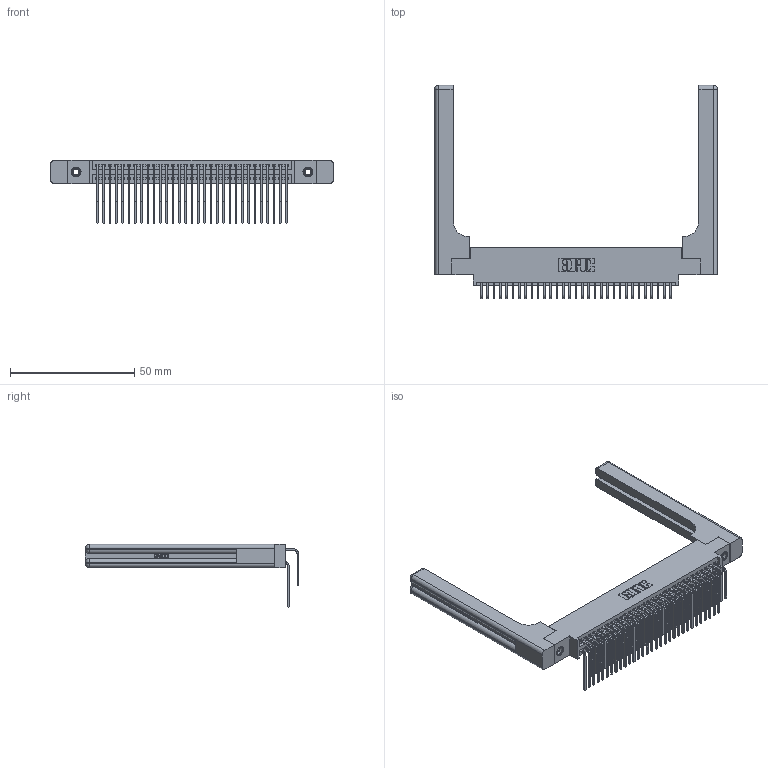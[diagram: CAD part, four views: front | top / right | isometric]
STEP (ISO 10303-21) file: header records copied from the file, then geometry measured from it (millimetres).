
FILE_DESCRIPTION (( 'STEP AP203' ), '1' );
FILE_NAME ('395-062-559-858.STEP', '2019-10-23T17:14:37', ( '' ), ( '' ), 'SwSTEP 2.0', 'SolidWorks 2016', '' );
FILE_SCHEMA (( 'CONFIG_CONTROL_DESIGN' ));
Length unit declared in the file: inch
Products named in the file (6): 345 Part_0.170 Offset - 0.156 Dia-TH; 345-292-001_558 559 Tail - 1; 345-292-001_559 Tail - 2; 345-250-001_345-250-001-102; 345-220-058_345-220-058; 395-062-559-858
Assembly tree (67 placements, depth 2):
  395-062-559-858
    345 Part_0.170 Offset - 0.156 Dia-TH
    345-292-001_558 559 Tail - 1  x31
    345-292-001_559 Tail - 2  x31
    345-250-001_345-250-001-102  x2
    345-220-058_345-220-058  x2
Bounding box: 113.77 x 85.84 x 25.53 mm (x, y, z)
Volume: 19668.7 mm3; surface area: 23217.1 mm2
Topology: 67 solids, 67 shells, 3610 faces, 10629 edges, 6982 vertices
Faces by surface type: plane 2402, cylinder 1148, bspline 36, cone 12, sphere 8, torus 4
Entity records: 32770 total; most frequent: CARTESIAN_POINT 6544, ORIENTED_EDGE 5224, DIRECTION 4688, EDGE_CURVE 2612, LINE 2224, VECTOR 2224, VERTEX_POINT 1730, AXIS2_PLACEMENT_3D 1232
